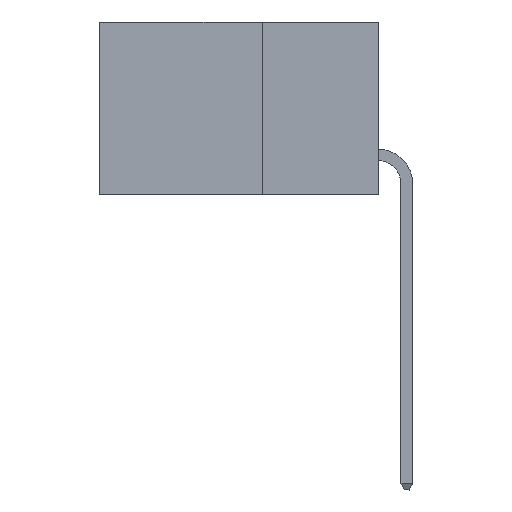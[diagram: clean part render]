
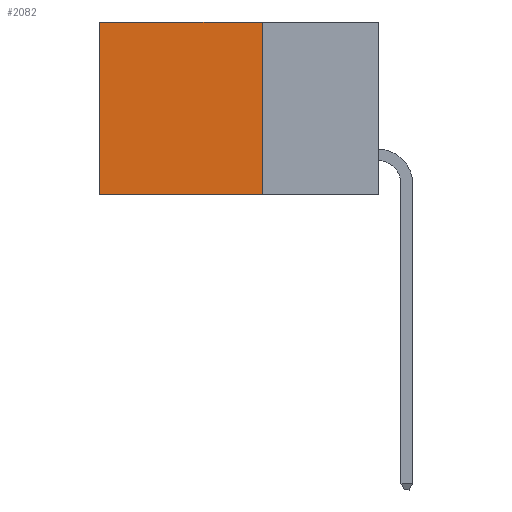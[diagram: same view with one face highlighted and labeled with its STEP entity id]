
A CAD part, left-side view. The second image highlights one B-rep face of the part: STEP entity #2082.
In plain terms, the highlighted planar face has unit normal (-1, 0, 0).
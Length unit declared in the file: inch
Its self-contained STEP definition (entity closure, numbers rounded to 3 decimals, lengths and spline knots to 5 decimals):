
#1097 = VECTOR ( 'NONE', #19042, 39.37008 ) ;
#2082 = ADVANCED_FACE ( 'NONE', ( #8701 ), #14625, .F. ) ;
#3173 = CARTESIAN_POINT ( 'NONE',  ( 0.298, 0.25, -0.37 ) ) ;
#3458 = CARTESIAN_POINT ( 'NONE',  ( 0.298, 0.25, 0. ) ) ;
#3517 = EDGE_LOOP ( 'NONE', ( #12579, #17441, #5088, #19874 ) ) ;
#4000 = CARTESIAN_POINT ( 'NONE',  ( 0.298, 0.6, 0. ) ) ;
#4164 = VECTOR ( 'NONE', #18773, 39.37008 ) ;
#5088 = ORIENTED_EDGE ( 'NONE', *, *, #13583, .F. ) ;
#5228 = DIRECTION ( 'NONE',  ( 0., 1., 0. ) ) ;
#5236 = VERTEX_POINT ( 'NONE', #8089 ) ;
#5662 = CARTESIAN_POINT ( 'NONE',  ( 0.298, 0.25, 0. ) ) ;
#5915 = VERTEX_POINT ( 'NONE', #3458 ) ;
#6701 = VECTOR ( 'NONE', #5228, 39.37008 ) ;
#6758 = VERTEX_POINT ( 'NONE', #18722 ) ;
#8005 = EDGE_CURVE ( 'NONE', #5236, #6758, #13749, .T. ) ;
#8089 = CARTESIAN_POINT ( 'NONE',  ( 0.298, 0.6, 0. ) ) ;
#8108 = LINE ( 'NONE', #14657, #19810 ) ;
#8701 = FACE_OUTER_BOUND ( 'NONE', #3517, .T. ) ;
#9214 = EDGE_CURVE ( 'NONE', #12505, #6758, #15526, .T. ) ;
#11136 = DIRECTION ( 'NONE',  ( 1., 0., 0. ) ) ;
#11570 = EDGE_CURVE ( 'NONE', #5915, #5236, #8108, .T. ) ;
#12505 = VERTEX_POINT ( 'NONE', #3173 ) ;
#12579 = ORIENTED_EDGE ( 'NONE', *, *, #8005, .T. ) ;
#13254 = CARTESIAN_POINT ( 'NONE',  ( 0.298, 0.25, -0.37 ) ) ;
#13583 = EDGE_CURVE ( 'NONE', #5915, #12505, #18150, .T. ) ;
#13749 = LINE ( 'NONE', #4000, #4164 ) ;
#14625 = PLANE ( 'NONE',  #18279 ) ;
#14657 = CARTESIAN_POINT ( 'NONE',  ( 0.298, 0.25, 0. ) ) ;
#14947 = DIRECTION ( 'NONE',  ( 0., 1., 0. ) ) ;
#15526 = LINE ( 'NONE', #13254, #6701 ) ;
#17441 = ORIENTED_EDGE ( 'NONE', *, *, #9214, .F. ) ;
#17873 = CARTESIAN_POINT ( 'NONE',  ( 0.298, 0.25, 0. ) ) ;
#18150 = LINE ( 'NONE', #5662, #1097 ) ;
#18279 = AXIS2_PLACEMENT_3D ( 'NONE', #17873, #11136, #19551 ) ;
#18722 = CARTESIAN_POINT ( 'NONE',  ( 0.298, 0.6, -0.37 ) ) ;
#18773 = DIRECTION ( 'NONE',  ( 0., 0., -1. ) ) ;
#19042 = DIRECTION ( 'NONE',  ( 0., 0., -1. ) ) ;
#19551 = DIRECTION ( 'NONE',  ( 0., 0., -1. ) ) ;
#19810 = VECTOR ( 'NONE', #14947, 39.37008 ) ;
#19874 = ORIENTED_EDGE ( 'NONE', *, *, #11570, .T. ) ;
